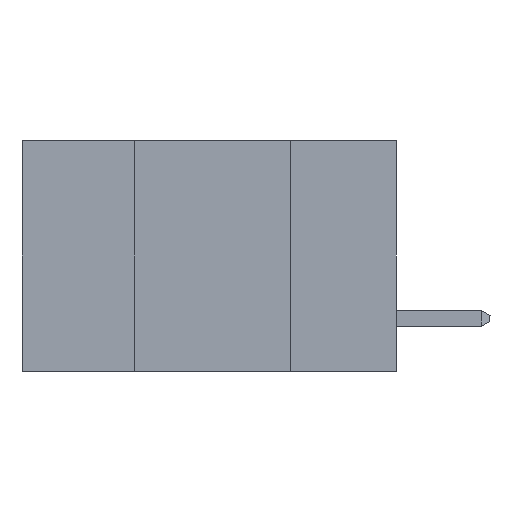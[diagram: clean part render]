
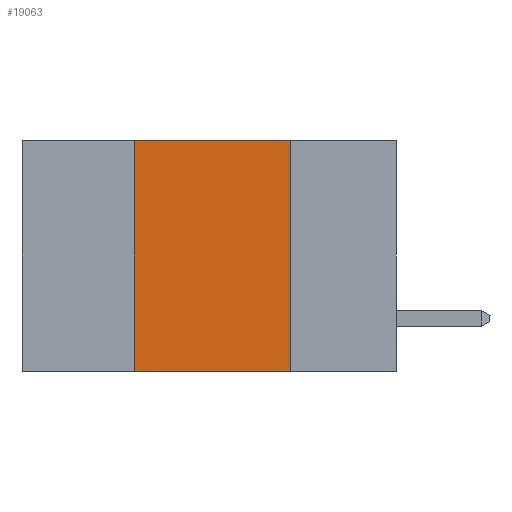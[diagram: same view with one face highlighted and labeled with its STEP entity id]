
A CAD part, left-side view. The second image highlights one B-rep face of the part: STEP entity #19063.
In plain terms, the highlighted planar face has unit normal (-1, 0, 0).
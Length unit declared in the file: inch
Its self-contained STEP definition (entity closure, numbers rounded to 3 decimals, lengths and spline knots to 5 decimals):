
#2803 = ORIENTED_EDGE ( 'NONE', *, *, #7280, .F. ) ;
#3892 = ORIENTED_EDGE ( 'NONE', *, *, #6679, .T. ) ;
#3896 = VERTEX_POINT ( 'NONE', #11809 ) ;
#5388 = DIRECTION ( 'NONE',  ( 1., 0., 0. ) ) ;
#5487 = CARTESIAN_POINT ( 'NONE',  ( 0., 0.17, 0. ) ) ;
#6122 = FACE_OUTER_BOUND ( 'NONE', #11201, .T. ) ;
#6677 = CARTESIAN_POINT ( 'NONE',  ( 0., 0.6, -0.37 ) ) ;
#6679 = EDGE_CURVE ( 'NONE', #3896, #21098, #17693, .T. ) ;
#7251 = VECTOR ( 'NONE', #15468, 39.37008 ) ;
#7272 = DIRECTION ( 'NONE',  ( 0., -1., 0. ) ) ;
#7280 = EDGE_CURVE ( 'NONE', #8794, #18566, #19945, .T. ) ;
#7402 = ORIENTED_EDGE ( 'NONE', *, *, #15634, .F. ) ;
#7637 = ORIENTED_EDGE ( 'NONE', *, *, #19369, .F. ) ;
#8189 = LINE ( 'NONE', #19789, #22094 ) ;
#8794 = VERTEX_POINT ( 'NONE', #9724 ) ;
#9064 = CARTESIAN_POINT ( 'NONE',  ( 0., 0.6, 0. ) ) ;
#9112 = VECTOR ( 'NONE', #22439, 39.37008 ) ;
#9210 = AXIS2_PLACEMENT_3D ( 'NONE', #9064, #5388, #18272 ) ;
#9222 = CARTESIAN_POINT ( 'NONE',  ( 0., 0.17, -0.37 ) ) ;
#9724 = CARTESIAN_POINT ( 'NONE',  ( 0., 0.42, 0. ) ) ;
#10926 = PLANE ( 'NONE',  #9210 ) ;
#11201 = EDGE_LOOP ( 'NONE', ( #7637, #2803, #7402, #3892 ) ) ;
#11809 = CARTESIAN_POINT ( 'NONE',  ( 0., 0.42, -0.37 ) ) ;
#15468 = DIRECTION ( 'NONE',  ( 0., 0., -1. ) ) ;
#15634 = EDGE_CURVE ( 'NONE', #3896, #8794, #8189, .T. ) ;
#17311 = CARTESIAN_POINT ( 'NONE',  ( 0., 0.17, -0.37 ) ) ;
#17693 = LINE ( 'NONE', #6677, #21852 ) ;
#18272 = DIRECTION ( 'NONE',  ( 0., 0., -1. ) ) ;
#18566 = VERTEX_POINT ( 'NONE', #5487 ) ;
#19063 = ADVANCED_FACE ( 'NONE', ( #6122 ), #10926, .F. ) ;
#19369 = EDGE_CURVE ( 'NONE', #18566, #21098, #21780, .T. ) ;
#19789 = CARTESIAN_POINT ( 'NONE',  ( 0., 0.42, -0.37 ) ) ;
#19945 = LINE ( 'NONE', #22331, #9112 ) ;
#21098 = VERTEX_POINT ( 'NONE', #9222 ) ;
#21531 = DIRECTION ( 'NONE',  ( 0., 0., 1. ) ) ;
#21780 = LINE ( 'NONE', #17311, #7251 ) ;
#21852 = VECTOR ( 'NONE', #7272, 39.37008 ) ;
#22094 = VECTOR ( 'NONE', #21531, 39.37008 ) ;
#22331 = CARTESIAN_POINT ( 'NONE',  ( 0., 0.6, 0. ) ) ;
#22439 = DIRECTION ( 'NONE',  ( 0., -1., 0. ) ) ;
